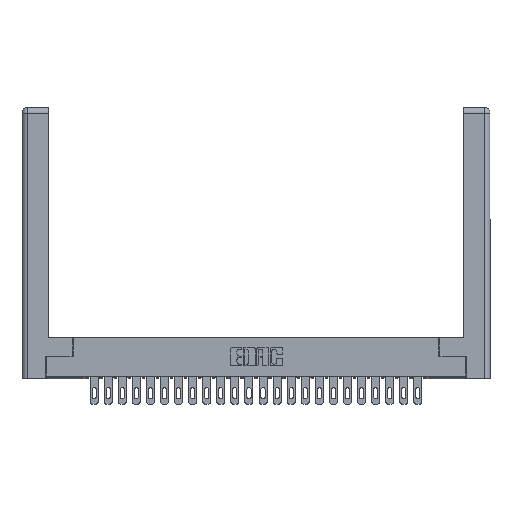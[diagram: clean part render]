
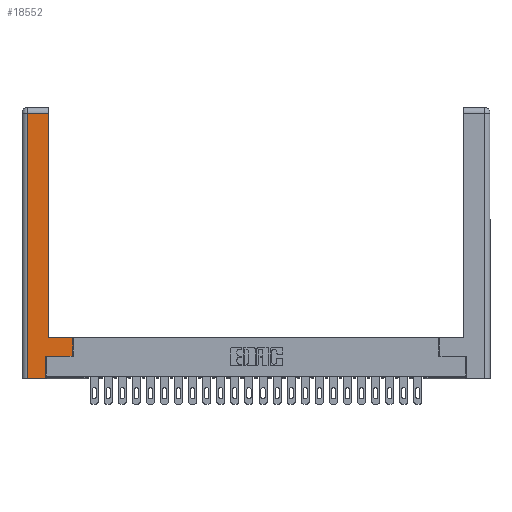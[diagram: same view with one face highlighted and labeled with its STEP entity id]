
A CAD part, top view. The second image highlights one B-rep face of the part: STEP entity #18552.
In plain terms, the highlighted planar face has unit normal (0, 0, 1).
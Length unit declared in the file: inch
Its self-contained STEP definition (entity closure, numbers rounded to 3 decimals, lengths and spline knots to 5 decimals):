
#711 = CARTESIAN_POINT ( 'NONE',  ( 0.0615, 2.94, 0. ) ) ;
#856 = LINE ( 'NONE', #3100, #23551 ) ;
#1011 = CARTESIAN_POINT ( 'NONE',  ( 0.0615, 0., 0. ) ) ;
#1122 = AXIS2_PLACEMENT_3D ( 'NONE', #3743, #10827, #27541 ) ;
#2030 = DIRECTION ( 'NONE',  ( -1., 0., 0. ) ) ;
#2131 = LINE ( 'NONE', #30431, #28517 ) ;
#2398 = CARTESIAN_POINT ( 'NONE',  ( 0.295, 2.94, 0. ) ) ;
#2474 = ORIENTED_EDGE ( 'NONE', *, *, #14083, .T. ) ;
#3100 = CARTESIAN_POINT ( 'NONE',  ( 0.0615, 2.94, 0. ) ) ;
#3564 = EDGE_CURVE ( 'NONE', #12421, #24363, #856, .T. ) ;
#3743 = CARTESIAN_POINT ( 'NONE',  ( 0., 0., 0. ) ) ;
#3772 = EDGE_CURVE ( 'NONE', #30309, #13713, #22781, .T. ) ;
#4348 = LINE ( 'NONE', #15123, #22610 ) ;
#5095 = VERTEX_POINT ( 'NONE', #14212 ) ;
#5637 = EDGE_LOOP ( 'NONE', ( #29005, #20609, #19825, #15203, #15427, #26717, #2474, #16953 ) ) ;
#5690 = DIRECTION ( 'NONE',  ( -1., 0., 0. ) ) ;
#6068 = CARTESIAN_POINT ( 'NONE',  ( 0.565, 0.245, 0. ) ) ;
#7785 = VERTEX_POINT ( 'NONE', #11083 ) ;
#8383 = LINE ( 'NONE', #1011, #9869 ) ;
#8524 = PLANE ( 'NONE',  #1122 ) ;
#8617 = CARTESIAN_POINT ( 'NONE',  ( 0.565, 0.45, 0. ) ) ;
#8710 = DIRECTION ( 'NONE',  ( 0., 1., 0. ) ) ;
#9869 = VECTOR ( 'NONE', #17635, 39.37008 ) ;
#10827 = DIRECTION ( 'NONE',  ( 0., 0., -1. ) ) ;
#11083 = CARTESIAN_POINT ( 'NONE',  ( 0.565, 0.45, 0. ) ) ;
#11360 = DIRECTION ( 'NONE',  ( 0., 1., 0. ) ) ;
#12421 = VERTEX_POINT ( 'NONE', #2398 ) ;
#12847 = EDGE_CURVE ( 'NONE', #7785, #5095, #2131, .T. ) ;
#13250 = LINE ( 'NONE', #8617, #16206 ) ;
#13713 = VERTEX_POINT ( 'NONE', #27191 ) ;
#14083 = EDGE_CURVE ( 'NONE', #13713, #7785, #13250, .T. ) ;
#14212 = CARTESIAN_POINT ( 'NONE',  ( 0.295, 0.45, 0. ) ) ;
#14466 = EDGE_CURVE ( 'NONE', #24363, #21297, #8383, .T. ) ;
#14810 = DIRECTION ( 'NONE',  ( 1., 0., 0. ) ) ;
#15118 = VECTOR ( 'NONE', #11360, 39.37008 ) ;
#15123 = CARTESIAN_POINT ( 'NONE',  ( 0.265, 0., 0. ) ) ;
#15203 = ORIENTED_EDGE ( 'NONE', *, *, #28311, .T. ) ;
#15328 = CARTESIAN_POINT ( 'NONE',  ( 0.265, 0., 0. ) ) ;
#15427 = ORIENTED_EDGE ( 'NONE', *, *, #25325, .T. ) ;
#15596 = DIRECTION ( 'NONE',  ( 0., 1., 0. ) ) ;
#15830 = CARTESIAN_POINT ( 'NONE',  ( 0.295, 3., 0. ) ) ;
#16206 = VECTOR ( 'NONE', #8710, 39.37008 ) ;
#16953 = ORIENTED_EDGE ( 'NONE', *, *, #12847, .T. ) ;
#17306 = VECTOR ( 'NONE', #15596, 39.37008 ) ;
#17635 = DIRECTION ( 'NONE',  ( 0., -1., 0. ) ) ;
#18240 = DIRECTION ( 'NONE',  ( 1., 0., 0. ) ) ;
#18447 = LINE ( 'NONE', #15830, #15118 ) ;
#18552 = ADVANCED_FACE ( 'NONE', ( #19716 ), #8524, .F. ) ;
#19073 = VERTEX_POINT ( 'NONE', #15328 ) ;
#19424 = VECTOR ( 'NONE', #18240, 39.37008 ) ;
#19716 = FACE_OUTER_BOUND ( 'NONE', #5637, .T. ) ;
#19825 = ORIENTED_EDGE ( 'NONE', *, *, #14466, .T. ) ;
#20137 = CARTESIAN_POINT ( 'NONE',  ( 0.265, 0.245, 0. ) ) ;
#20609 = ORIENTED_EDGE ( 'NONE', *, *, #3564, .T. ) ;
#21297 = VERTEX_POINT ( 'NONE', #23564 ) ;
#22610 = VECTOR ( 'NONE', #14810, 39.37008 ) ;
#22781 = LINE ( 'NONE', #6068, #19424 ) ;
#23551 = VECTOR ( 'NONE', #5690, 39.37008 ) ;
#23564 = CARTESIAN_POINT ( 'NONE',  ( 0.0615, 0., 0. ) ) ;
#24363 = VERTEX_POINT ( 'NONE', #711 ) ;
#24872 = CARTESIAN_POINT ( 'NONE',  ( 0.265, 0.245, 0. ) ) ;
#24968 = EDGE_CURVE ( 'NONE', #5095, #12421, #18447, .T. ) ;
#25134 = LINE ( 'NONE', #24872, #17306 ) ;
#25325 = EDGE_CURVE ( 'NONE', #19073, #30309, #25134, .T. ) ;
#26717 = ORIENTED_EDGE ( 'NONE', *, *, #3772, .T. ) ;
#27191 = CARTESIAN_POINT ( 'NONE',  ( 0.565, 0.245, 0. ) ) ;
#27541 = DIRECTION ( 'NONE',  ( -1., 0., 0. ) ) ;
#28311 = EDGE_CURVE ( 'NONE', #21297, #19073, #4348, .T. ) ;
#28517 = VECTOR ( 'NONE', #2030, 39.37008 ) ;
#29005 = ORIENTED_EDGE ( 'NONE', *, *, #24968, .T. ) ;
#30309 = VERTEX_POINT ( 'NONE', #20137 ) ;
#30431 = CARTESIAN_POINT ( 'NONE',  ( 0.295, 0.45, 0. ) ) ;
